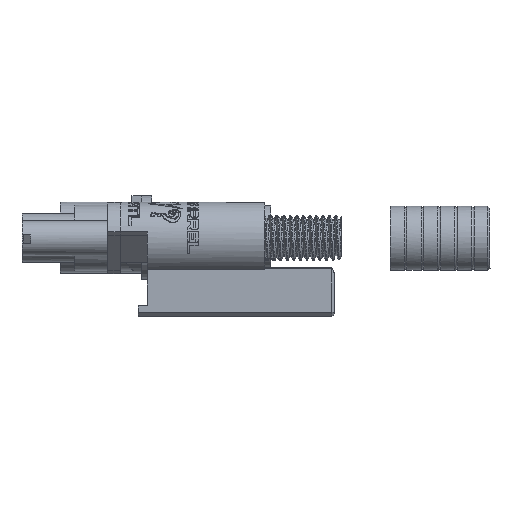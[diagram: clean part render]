
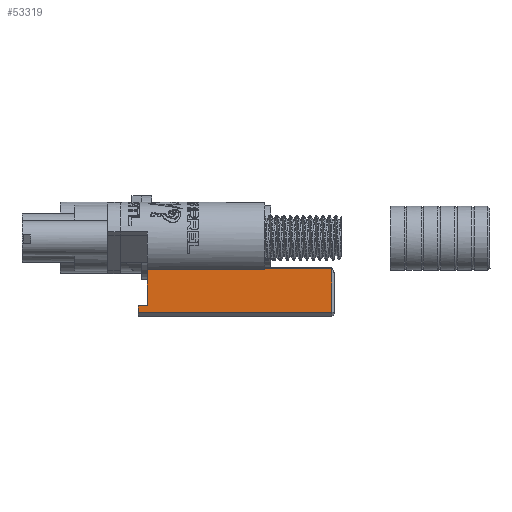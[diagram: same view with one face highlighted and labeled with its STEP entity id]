
A CAD part, left-side view. The second image highlights one B-rep face of the part: STEP entity #53319.
In plain terms, the highlighted planar face has unit normal (-1, 0, 0).
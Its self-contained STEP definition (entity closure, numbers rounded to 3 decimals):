
#2239=PLANE('',#56466);
#3153=FACE_OUTER_BOUND('',#6238,.T.);
#6238=EDGE_LOOP('',(#36991,#36992,#36993,#36994,#36995,#36996,#36997,#36998));
#14752=LINE('',#70364,#18065);
#14796=LINE('',#73259,#18109);
#14799=LINE('',#73265,#18112);
#14802=LINE('',#73271,#18115);
#14803=LINE('',#73272,#18116);
#14804=LINE('',#73274,#18117);
#14805=LINE('',#73276,#18118);
#14806=LINE('',#73277,#18119);
#18065=VECTOR('',#58477,10.);
#18109=VECTOR('',#58593,10.);
#18112=VECTOR('',#58600,10.);
#18115=VECTOR('',#58605,10.);
#18116=VECTOR('',#58606,10.);
#18117=VECTOR('',#58607,10.);
#18118=VECTOR('',#58608,10.);
#18119=VECTOR('',#58609,10.);
#21504=VERTEX_POINT('',#70350);
#21510=VERTEX_POINT('',#70362);
#21978=VERTEX_POINT('',#73134);
#21982=VERTEX_POINT('',#73216);
#21985=VERTEX_POINT('',#73264);
#21987=VERTEX_POINT('',#73270);
#21988=VERTEX_POINT('',#73273);
#21989=VERTEX_POINT('',#73275);
#27412=EDGE_CURVE('',#21504,#21510,#14752,.T.);
#27898=EDGE_CURVE('',#21982,#21978,#14796,.T.);
#27901=EDGE_CURVE('',#21978,#21985,#14799,.F.);
#27904=EDGE_CURVE('',#21982,#21987,#14802,.T.);
#27905=EDGE_CURVE('',#21987,#21504,#14803,.F.);
#27906=EDGE_CURVE('',#21510,#21988,#14804,.T.);
#27907=EDGE_CURVE('',#21989,#21988,#14805,.F.);
#27908=EDGE_CURVE('',#21989,#21985,#14806,.T.);
#36991=ORIENTED_EDGE('',*,*,#27898,.F.);
#36992=ORIENTED_EDGE('',*,*,#27904,.T.);
#36993=ORIENTED_EDGE('',*,*,#27905,.T.);
#36994=ORIENTED_EDGE('',*,*,#27412,.T.);
#36995=ORIENTED_EDGE('',*,*,#27906,.T.);
#36996=ORIENTED_EDGE('',*,*,#27907,.F.);
#36997=ORIENTED_EDGE('',*,*,#27908,.T.);
#36998=ORIENTED_EDGE('',*,*,#27901,.F.);
#53319=ADVANCED_FACE('',(#3153),#2239,.T.);
#56466=AXIS2_PLACEMENT_3D('',#73269,#58603,#58604);
#58477=DIRECTION('',(0.,1.,0.));
#58593=DIRECTION('',(0.,0.,-1.));
#58600=DIRECTION('',(0.,-1.,0.));
#58603=DIRECTION('center_axis',(-1.,0.,0.));
#58604=DIRECTION('ref_axis',(0.,0.,
1.));
#58605=DIRECTION('',(0.,1.,0.));
#58606=DIRECTION('',(0.,0.,1.));
#58607=DIRECTION('',(0.,0.,-1.));
#58608=DIRECTION('',(0.,0.999,-0.037));
#58609=DIRECTION('',(0.,0.,-1.));
#70350=CARTESIAN_POINT('',(-766.129,-158.345,-10.084));
#70362=CARTESIAN_POINT('',(-766.126,-116.599,-10.086));
#70364=CARTESIAN_POINT('',(-766.126,-116.599,-10.086));
#73134=CARTESIAN_POINT('',(-766.131,-182.2,-25.352));
#73216=CARTESIAN_POINT('',(-766.131,-182.199,-9.772));
#73259=CARTESIAN_POINT('',(-766.131,-182.199,-6.187));
#73264=CARTESIAN_POINT('',(-766.126,-113.35,-25.355));
#73265=CARTESIAN_POINT('',(-766.129,-156.475,-25.353));
#73269=CARTESIAN_POINT('Origin',(-766.128,-149.899,-10.721));
#73270=CARTESIAN_POINT('',(-766.129,-158.345,-9.773));
#73271=CARTESIAN_POINT('',(-766.131,-183.199,-9.772));
#73272=CARTESIAN_POINT('',(-766.129,-158.345,-13.989));
#73273=CARTESIAN_POINT('',(-766.126,-116.6,-22.835));
#73274=CARTESIAN_POINT('',(-766.126,-116.599,-10.722));
#73275=CARTESIAN_POINT('',(-766.126,-113.35,-22.956));
#73276=CARTESIAN_POINT('',(-766.127,-133.44,-22.208));
#73277=CARTESIAN_POINT('',(-766.126,-113.349,-10.723));
